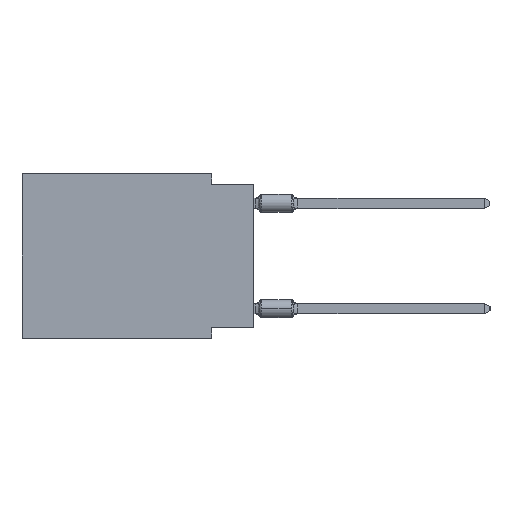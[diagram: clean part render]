
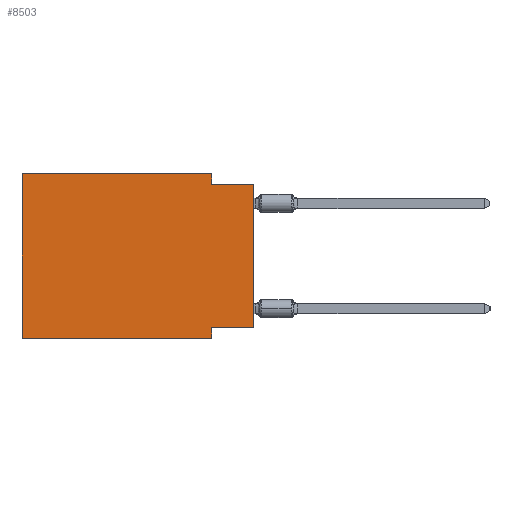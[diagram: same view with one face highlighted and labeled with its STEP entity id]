
A CAD part, left-side view. The second image highlights one B-rep face of the part: STEP entity #8503.
In plain terms, the highlighted planar face has unit normal (-1, 0, 0).
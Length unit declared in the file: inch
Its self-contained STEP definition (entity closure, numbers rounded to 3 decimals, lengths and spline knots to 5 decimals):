
#425 = VECTOR ( 'NONE', #32411, 39.37008 ) ;
#454 = LINE ( 'NONE', #38430, #17244 ) ;
#475 = LINE ( 'NONE', #10027, #5132 ) ;
#647 = LINE ( 'NONE', #16417, #425 ) ;
#688 = DIRECTION ( 'NONE',  ( 0., -1., 0. ) ) ;
#1898 = CARTESIAN_POINT ( 'NONE',  ( 0., 0., -0.365 ) ) ;
#1975 = VERTEX_POINT ( 'NONE', #14435 ) ;
#2752 = EDGE_CURVE ( 'NONE', #24140, #39467, #454, .T. ) ;
#4321 = CARTESIAN_POINT ( 'NONE',  ( 0., 0.1, -0.39 ) ) ;
#5116 = DIRECTION ( 'NONE',  ( 0., -1., 0. ) ) ;
#5132 = VECTOR ( 'NONE', #688, 39.37008 ) ;
#5514 = DIRECTION ( 'NONE',  ( 0., 0., 1. ) ) ;
#5620 = CARTESIAN_POINT ( 'NONE',  ( 0., 0.1, -0.365 ) ) ;
#5639 = CARTESIAN_POINT ( 'NONE',  ( 0., 0.1, 0. ) ) ;
#6536 = AXIS2_PLACEMENT_3D ( 'NONE', #33452, #14778, #32860 ) ;
#7489 = ORIENTED_EDGE ( 'NONE', *, *, #15970, .F. ) ;
#7516 = ORIENTED_EDGE ( 'NONE', *, *, #17934, .F. ) ;
#8503 = ADVANCED_FACE ( 'NONE', ( #30151 ), #14168, .F. ) ;
#9045 = CARTESIAN_POINT ( 'NONE',  ( 0., 0.55, 0. ) ) ;
#10027 = CARTESIAN_POINT ( 'NONE',  ( 0., 0., -0.025 ) ) ;
#10107 = CARTESIAN_POINT ( 'NONE',  ( 0., 0., -0.365 ) ) ;
#10498 = VERTEX_POINT ( 'NONE', #4321 ) ;
#10591 = EDGE_CURVE ( 'NONE', #37922, #10498, #32981, .T. ) ;
#12871 = CARTESIAN_POINT ( 'NONE',  ( 0., 0.55, -0.39 ) ) ;
#13116 = DIRECTION ( 'NONE',  ( 0., 0., 1. ) ) ;
#13184 = VECTOR ( 'NONE', #5116, 39.37008 ) ;
#14168 = PLANE ( 'NONE',  #6536 ) ;
#14435 = CARTESIAN_POINT ( 'NONE',  ( 0., 0.1, -0.025 ) ) ;
#14778 = DIRECTION ( 'NONE',  ( 1., 0., 0. ) ) ;
#15547 = ORIENTED_EDGE ( 'NONE', *, *, #2752, .T. ) ;
#15615 = DIRECTION ( 'NONE',  ( 0., 0., -1. ) ) ;
#15657 = ORIENTED_EDGE ( 'NONE', *, *, #21545, .F. ) ;
#15970 = EDGE_CURVE ( 'NONE', #40011, #10498, #17920, .T. ) ;
#16162 = CARTESIAN_POINT ( 'NONE',  ( 0., 0., -0.025 ) ) ;
#16417 = CARTESIAN_POINT ( 'NONE',  ( 0., 0.55, 0. ) ) ;
#16830 = EDGE_CURVE ( 'NONE', #37922, #27537, #27961, .T. ) ;
#17244 = VECTOR ( 'NONE', #13116, 39.37008 ) ;
#17920 = LINE ( 'NONE', #27277, #26162 ) ;
#17934 = EDGE_CURVE ( 'NONE', #27537, #28268, #647, .T. ) ;
#18747 = ORIENTED_EDGE ( 'NONE', *, *, #16830, .F. ) ;
#19978 = ORIENTED_EDGE ( 'NONE', *, *, #10591, .T. ) ;
#21545 = EDGE_CURVE ( 'NONE', #1975, #39467, #475, .T. ) ;
#21589 = VECTOR ( 'NONE', #5514, 39.37008 ) ;
#21666 = EDGE_LOOP ( 'NONE', ( #15547, #15657, #30985, #7516, #18747, #19978, #7489, #38175 ) ) ;
#22265 = VECTOR ( 'NONE', #15615, 39.37008 ) ;
#22787 = DIRECTION ( 'NONE',  ( 0., 1., 0. ) ) ;
#24140 = VERTEX_POINT ( 'NONE', #1898 ) ;
#24367 = DIRECTION ( 'NONE',  ( 0., 0., -1. ) ) ;
#26162 = VECTOR ( 'NONE', #24367, 39.37008 ) ;
#27277 = CARTESIAN_POINT ( 'NONE',  ( 0., 0.1, -0.39 ) ) ;
#27537 = VERTEX_POINT ( 'NONE', #27630 ) ;
#27630 = CARTESIAN_POINT ( 'NONE',  ( 0., 0.55, 0. ) ) ;
#27961 = LINE ( 'NONE', #9045, #21589 ) ;
#28268 = VERTEX_POINT ( 'NONE', #35876 ) ;
#29825 = LINE ( 'NONE', #10107, #35988 ) ;
#30151 = FACE_OUTER_BOUND ( 'NONE', #21666, .T. ) ;
#30783 = LINE ( 'NONE', #5639, #22265 ) ;
#30985 = ORIENTED_EDGE ( 'NONE', *, *, #37261, .F. ) ;
#31579 = EDGE_CURVE ( 'NONE', #24140, #40011, #29825, .T. ) ;
#32411 = DIRECTION ( 'NONE',  ( 0., -1., 0. ) ) ;
#32860 = DIRECTION ( 'NONE',  ( 0., 0., -1. ) ) ;
#32981 = LINE ( 'NONE', #33578, #13184 ) ;
#33452 = CARTESIAN_POINT ( 'NONE',  ( 0., 0.55, 0. ) ) ;
#33578 = CARTESIAN_POINT ( 'NONE',  ( 0., 0.55, -0.39 ) ) ;
#35876 = CARTESIAN_POINT ( 'NONE',  ( 0., 0.1, 0. ) ) ;
#35988 = VECTOR ( 'NONE', #22787, 39.37008 ) ;
#37261 = EDGE_CURVE ( 'NONE', #28268, #1975, #30783, .T. ) ;
#37922 = VERTEX_POINT ( 'NONE', #12871 ) ;
#38175 = ORIENTED_EDGE ( 'NONE', *, *, #31579, .F. ) ;
#38430 = CARTESIAN_POINT ( 'NONE',  ( 0., 0., 0. ) ) ;
#39467 = VERTEX_POINT ( 'NONE', #16162 ) ;
#40011 = VERTEX_POINT ( 'NONE', #5620 ) ;
